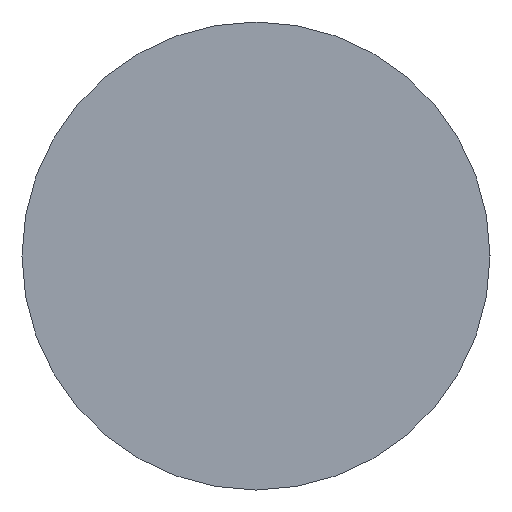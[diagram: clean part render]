
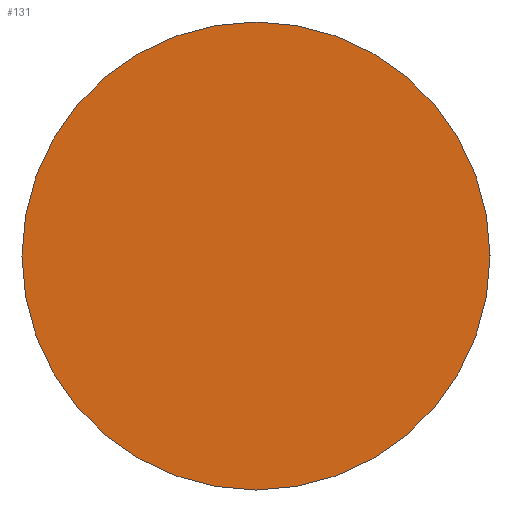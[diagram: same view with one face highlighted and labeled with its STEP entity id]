
A CAD part, left-side view. The second image highlights one B-rep face of the part: STEP entity #131.
In plain terms, the highlighted planar face has unit normal (-1, 0, 0).
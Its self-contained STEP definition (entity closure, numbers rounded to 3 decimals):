
#10 = EDGE_LOOP ( 'NONE', ( #101, #122 ) ) ;
#13 = DIRECTION ( 'NONE',  ( 0., 0., -1. ) ) ;
#20 = CARTESIAN_POINT ( 'NONE',  ( 0., 0., 0. ) ) ;
#21 = AXIS2_PLACEMENT_3D ( 'NONE', #116, #109, #89 ) ;
#34 = DIRECTION ( 'NONE',  ( 1., 0., 0. ) ) ;
#35 = EDGE_CURVE ( 'NONE', #107, #118, #68, .T. ) ;
#37 = CIRCLE ( 'NONE', #80, 1.588 ) ;
#44 = EDGE_CURVE ( 'NONE', #118, #107, #37, .T. ) ;
#51 = CARTESIAN_POINT ( 'NONE',  ( 0., 0., 1.588 ) ) ;
#64 = CARTESIAN_POINT ( 'NONE',  ( 0., 0., 0. ) ) ;
#68 = CIRCLE ( 'NONE', #97, 1.588 ) ;
#80 = AXIS2_PLACEMENT_3D ( 'NONE', #20, #86, #13 ) ;
#85 = FACE_OUTER_BOUND ( 'NONE', #10, .T. ) ;
#86 = DIRECTION ( 'NONE',  ( 1., 0., 0. ) ) ;
#89 = DIRECTION ( 'NONE',  ( 0., 0., -1. ) ) ;
#94 = DIRECTION ( 'NONE',  ( 0., 0., -1. ) ) ;
#97 = AXIS2_PLACEMENT_3D ( 'NONE', #64, #34, #94 ) ;
#101 = ORIENTED_EDGE ( 'NONE', *, *, #35, .F. ) ;
#107 = VERTEX_POINT ( 'NONE', #51 ) ;
#109 = DIRECTION ( 'NONE',  ( 1., 0., 0. ) ) ;
#111 = PLANE ( 'NONE',  #21 ) ;
#116 = CARTESIAN_POINT ( 'NONE',  ( 0., 0., 0. ) ) ;
#117 = CARTESIAN_POINT ( 'NONE',  ( 0., 0., -1.588 ) ) ;
#118 = VERTEX_POINT ( 'NONE', #117 ) ;
#122 = ORIENTED_EDGE ( 'NONE', *, *, #44, .F. ) ;
#131 = ADVANCED_FACE ( 'NONE', ( #85 ), #111, .F. ) ;
